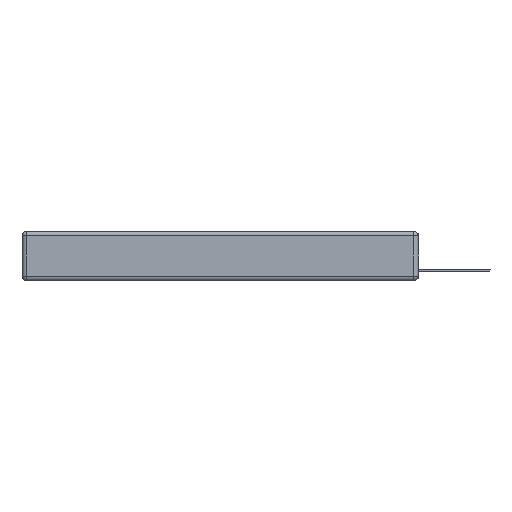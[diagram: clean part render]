
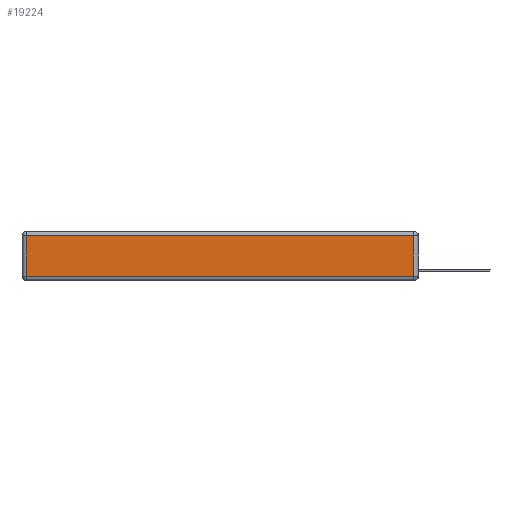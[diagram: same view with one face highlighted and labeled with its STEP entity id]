
A CAD part, left-side view. The second image highlights one B-rep face of the part: STEP entity #19224.
In plain terms, the highlighted planar face has unit normal (-1, 0, 0).
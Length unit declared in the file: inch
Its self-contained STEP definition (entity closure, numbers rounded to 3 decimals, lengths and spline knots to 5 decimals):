
#1178 = CARTESIAN_POINT ( 'NONE',  ( 0., 2.75, -0.03 ) ) ;
#1209 = ORIENTED_EDGE ( 'NONE', *, *, #18034, .T. ) ;
#1218 = VERTEX_POINT ( 'NONE', #1831 ) ;
#1351 = LINE ( 'NONE', #3202, #16615 ) ;
#1794 = CARTESIAN_POINT ( 'NONE',  ( 0., 0.03, -0.343 ) ) ;
#1831 = CARTESIAN_POINT ( 'NONE',  ( 0., 0.03, -0.03 ) ) ;
#2664 = VERTEX_POINT ( 'NONE', #4631 ) ;
#2892 = DIRECTION ( 'NONE',  ( 0., 1., 0. ) ) ;
#3091 = FACE_OUTER_BOUND ( 'NONE', #4163, .T. ) ;
#3202 = CARTESIAN_POINT ( 'NONE',  ( 0., 2.72, -0.343 ) ) ;
#3909 = CARTESIAN_POINT ( 'NONE',  ( 0., 0., -0.313 ) ) ;
#4163 = EDGE_LOOP ( 'NONE', ( #18336, #1209, #18003, #16233 ) ) ;
#4299 = EDGE_CURVE ( 'NONE', #2664, #7829, #1351, .T. ) ;
#4631 = CARTESIAN_POINT ( 'NONE',  ( 0., 2.72, -0.03 ) ) ;
#6441 = EDGE_CURVE ( 'NONE', #1218, #2664, #17523, .T. ) ;
#6734 = DIRECTION ( 'NONE',  ( -1., 0., 0. ) ) ;
#6811 = DIRECTION ( 'NONE',  ( 0., 0., 1. ) ) ;
#7829 = VERTEX_POINT ( 'NONE', #22487 ) ;
#8801 = DIRECTION ( 'NONE',  ( 0., 0., -1. ) ) ;
#8957 = VERTEX_POINT ( 'NONE', #13669 ) ;
#10562 = EDGE_CURVE ( 'NONE', #7829, #8957, #22404, .T. ) ;
#12337 = PLANE ( 'NONE',  #14584 ) ;
#12904 = VECTOR ( 'NONE', #2892, 39.37008 ) ;
#13669 = CARTESIAN_POINT ( 'NONE',  ( 0., 0.03, -0.313 ) ) ;
#14301 = CARTESIAN_POINT ( 'NONE',  ( 0., 0., -0.343 ) ) ;
#14584 = AXIS2_PLACEMENT_3D ( 'NONE', #14301, #6734, #20002 ) ;
#15703 = VECTOR ( 'NONE', #6811, 39.37008 ) ;
#15706 = VECTOR ( 'NONE', #24005, 39.37008 ) ;
#16233 = ORIENTED_EDGE ( 'NONE', *, *, #4299, .T. ) ;
#16315 = LINE ( 'NONE', #1794, #15703 ) ;
#16615 = VECTOR ( 'NONE', #8801, 39.37008 ) ;
#17523 = LINE ( 'NONE', #1178, #12904 ) ;
#18003 = ORIENTED_EDGE ( 'NONE', *, *, #6441, .T. ) ;
#18034 = EDGE_CURVE ( 'NONE', #8957, #1218, #16315, .T. ) ;
#18336 = ORIENTED_EDGE ( 'NONE', *, *, #10562, .T. ) ;
#19224 = ADVANCED_FACE ( 'NONE', ( #3091 ), #12337, .T. ) ;
#20002 = DIRECTION ( 'NONE',  ( 0., 0., 1. ) ) ;
#22404 = LINE ( 'NONE', #3909, #15706 ) ;
#22487 = CARTESIAN_POINT ( 'NONE',  ( 0., 2.72, -0.313 ) ) ;
#24005 = DIRECTION ( 'NONE',  ( 0., -1., 0. ) ) ;
